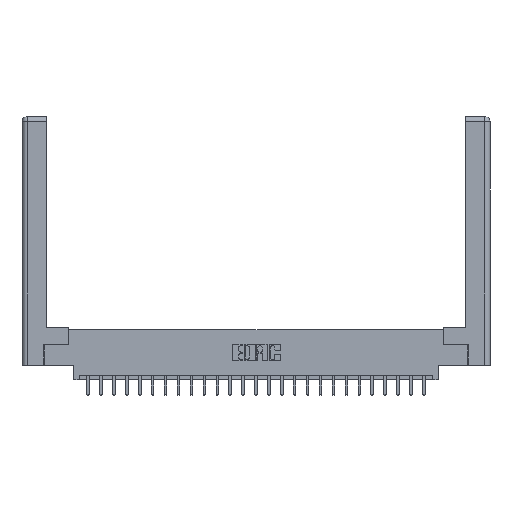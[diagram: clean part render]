
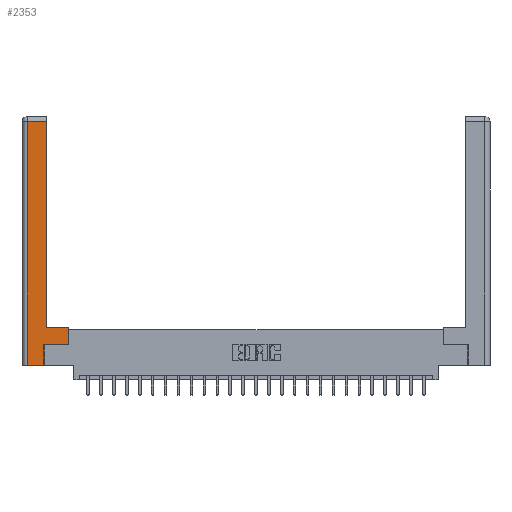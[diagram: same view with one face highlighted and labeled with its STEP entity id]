
A CAD part, top view. The second image highlights one B-rep face of the part: STEP entity #2353.
In plain terms, the highlighted planar face has unit normal (0, 0, 1).
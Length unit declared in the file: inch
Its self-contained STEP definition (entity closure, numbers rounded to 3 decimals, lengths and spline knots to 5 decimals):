
#429 = CARTESIAN_POINT ( 'NONE',  ( 0.265, 0.245, 0. ) ) ;
#1587 = VECTOR ( 'NONE', #14825, 39.37008 ) ;
#1693 = LINE ( 'NONE', #14425, #18864 ) ;
#2077 = VECTOR ( 'NONE', #21244, 39.37008 ) ;
#2353 = ADVANCED_FACE ( 'NONE', ( #4670 ), #5275, .F. ) ;
#4625 = VERTEX_POINT ( 'NONE', #14629 ) ;
#4670 = FACE_OUTER_BOUND ( 'NONE', #22369, .T. ) ;
#4891 = DIRECTION ( 'NONE',  ( 1., 0., 0. ) ) ;
#5275 = PLANE ( 'NONE',  #6458 ) ;
#5318 = CARTESIAN_POINT ( 'NONE',  ( 0.265, 0., 0. ) ) ;
#5628 = ORIENTED_EDGE ( 'NONE', *, *, #12237, .T. ) ;
#6227 = VERTEX_POINT ( 'NONE', #20590 ) ;
#6458 = AXIS2_PLACEMENT_3D ( 'NONE', #9087, #25041, #13099 ) ;
#6636 = EDGE_CURVE ( 'NONE', #25326, #12300, #23719, .T. ) ;
#6911 = VERTEX_POINT ( 'NONE', #429 ) ;
#7075 = LINE ( 'NONE', #11219, #2077 ) ;
#7894 = ORIENTED_EDGE ( 'NONE', *, *, #6636, .T. ) ;
#8323 = CARTESIAN_POINT ( 'NONE',  ( 0.295, 0.45, 0. ) ) ;
#8936 = EDGE_CURVE ( 'NONE', #18070, #6227, #15521, .T. ) ;
#9087 = CARTESIAN_POINT ( 'NONE',  ( 0., 0., 0. ) ) ;
#9383 = LINE ( 'NONE', #8323, #20656 ) ;
#10173 = ORIENTED_EDGE ( 'NONE', *, *, #17657, .T. ) ;
#10502 = DIRECTION ( 'NONE',  ( -1., 0., 0. ) ) ;
#11028 = VECTOR ( 'NONE', #12918, 39.37008 ) ;
#11080 = DIRECTION ( 'NONE',  ( 1., 0., 0. ) ) ;
#11198 = DIRECTION ( 'NONE',  ( -1., 0., 0. ) ) ;
#11219 = CARTESIAN_POINT ( 'NONE',  ( 0.265, 0.245, 0. ) ) ;
#12237 = EDGE_CURVE ( 'NONE', #12300, #18070, #24652, .T. ) ;
#12300 = VERTEX_POINT ( 'NONE', #25154 ) ;
#12388 = VECTOR ( 'NONE', #4891, 39.37008 ) ;
#12918 = DIRECTION ( 'NONE',  ( 0., 1., 0. ) ) ;
#12953 = LINE ( 'NONE', #18847, #11028 ) ;
#13099 = DIRECTION ( 'NONE',  ( -1., 0., 0. ) ) ;
#13127 = VECTOR ( 'NONE', #11198, 39.37008 ) ;
#13794 = VERTEX_POINT ( 'NONE', #19433 ) ;
#14311 = EDGE_CURVE ( 'NONE', #6227, #6911, #7075, .T. ) ;
#14425 = CARTESIAN_POINT ( 'NONE',  ( 0.295, 3., 0. ) ) ;
#14629 = CARTESIAN_POINT ( 'NONE',  ( 0.295, 0.45, 0. ) ) ;
#14825 = DIRECTION ( 'NONE',  ( 0., -1., 0. ) ) ;
#15521 = LINE ( 'NONE', #5318, #22685 ) ;
#15863 = ORIENTED_EDGE ( 'NONE', *, *, #8936, .T. ) ;
#16465 = CARTESIAN_POINT ( 'NONE',  ( 0.295, 2.94, 0. ) ) ;
#17262 = CARTESIAN_POINT ( 'NONE',  ( 0.0615, 2.94, 0. ) ) ;
#17657 = EDGE_CURVE ( 'NONE', #13794, #4625, #9383, .T. ) ;
#18070 = VERTEX_POINT ( 'NONE', #20680 ) ;
#18506 = EDGE_CURVE ( 'NONE', #20078, #13794, #12953, .T. ) ;
#18632 = EDGE_CURVE ( 'NONE', #6911, #20078, #22413, .T. ) ;
#18847 = CARTESIAN_POINT ( 'NONE',  ( 0.565, 0.45, 0. ) ) ;
#18864 = VECTOR ( 'NONE', #24440, 39.37008 ) ;
#19131 = CARTESIAN_POINT ( 'NONE',  ( 0.565, 0.245, 0. ) ) ;
#19327 = ORIENTED_EDGE ( 'NONE', *, *, #22160, .T. ) ;
#19433 = CARTESIAN_POINT ( 'NONE',  ( 0.565, 0.45, 0. ) ) ;
#19583 = ORIENTED_EDGE ( 'NONE', *, *, #18506, .T. ) ;
#20078 = VERTEX_POINT ( 'NONE', #19131 ) ;
#20181 = ORIENTED_EDGE ( 'NONE', *, *, #18632, .T. ) ;
#20590 = CARTESIAN_POINT ( 'NONE',  ( 0.265, 0., 0. ) ) ;
#20656 = VECTOR ( 'NONE', #10502, 39.37008 ) ;
#20680 = CARTESIAN_POINT ( 'NONE',  ( 0.0615, 0., 0. ) ) ;
#20908 = CARTESIAN_POINT ( 'NONE',  ( 0.0615, 0., 0. ) ) ;
#21193 = CARTESIAN_POINT ( 'NONE',  ( 0.565, 0.245, 0. ) ) ;
#21244 = DIRECTION ( 'NONE',  ( 0., 1., 0. ) ) ;
#22160 = EDGE_CURVE ( 'NONE', #4625, #25326, #1693, .T. ) ;
#22369 = EDGE_LOOP ( 'NONE', ( #19327, #7894, #5628, #15863, #23884, #20181, #19583, #10173 ) ) ;
#22413 = LINE ( 'NONE', #21193, #12388 ) ;
#22685 = VECTOR ( 'NONE', #11080, 39.37008 ) ;
#23719 = LINE ( 'NONE', #17262, #13127 ) ;
#23884 = ORIENTED_EDGE ( 'NONE', *, *, #14311, .T. ) ;
#24440 = DIRECTION ( 'NONE',  ( 0., 1., 0. ) ) ;
#24652 = LINE ( 'NONE', #20908, #1587 ) ;
#25041 = DIRECTION ( 'NONE',  ( 0., 0., -1. ) ) ;
#25154 = CARTESIAN_POINT ( 'NONE',  ( 0.0615, 2.94, 0. ) ) ;
#25326 = VERTEX_POINT ( 'NONE', #16465 ) ;
